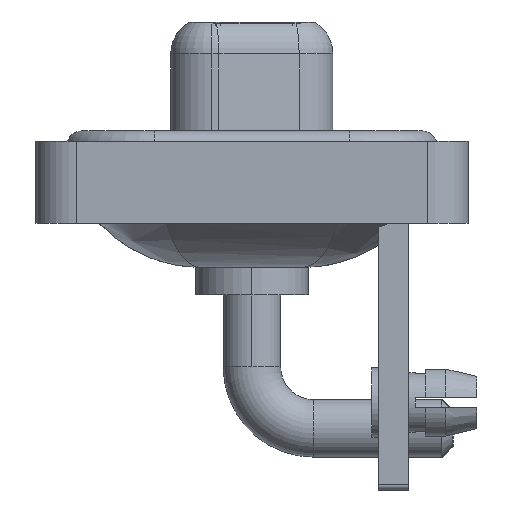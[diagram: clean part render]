
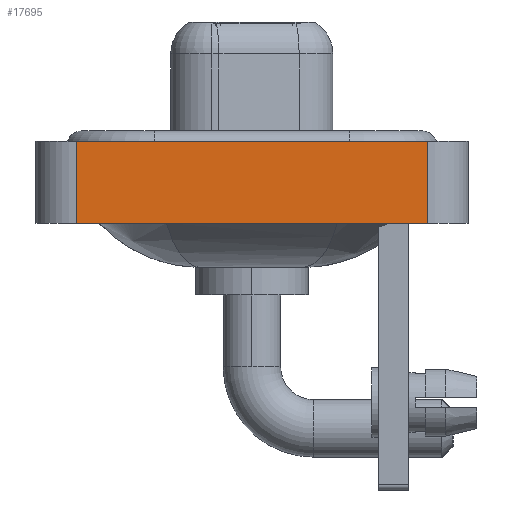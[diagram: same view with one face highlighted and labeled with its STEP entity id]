
A CAD part, left-side view. The second image highlights one B-rep face of the part: STEP entity #17695.
In plain terms, the highlighted planar face has unit normal (-1, 0, 0).
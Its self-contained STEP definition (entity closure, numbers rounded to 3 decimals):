
#284 = VERTEX_POINT ( 'NONE', #9182 ) ;
#681 = ORIENTED_EDGE ( 'NONE', *, *, #9010, .T. ) ;
#1089 = VERTEX_POINT ( 'NONE', #16234 ) ;
#1269 = VERTEX_POINT ( 'NONE', #14021 ) ;
#1744 = CARTESIAN_POINT ( 'NONE',  ( -7.3, 8.55, -3.6 ) ) ;
#1840 = ORIENTED_EDGE ( 'NONE', *, *, #10058, .F. ) ;
#1850 = EDGE_CURVE ( 'NONE', #13147, #1089, #11886, .T. ) ;
#1925 = LINE ( 'NONE', #2033, #12495 ) ;
#2018 = LINE ( 'NONE', #9761, #18036 ) ;
#2033 = CARTESIAN_POINT ( 'NONE',  ( -7.3, -8.55, -3.6 ) ) ;
#2707 = FACE_OUTER_BOUND ( 'NONE', #12504, .T. ) ;
#2946 = ORIENTED_EDGE ( 'NONE', *, *, #1850, .T. ) ;
#3979 = LINE ( 'NONE', #10131, #13502 ) ;
#5917 = EDGE_CURVE ( 'NONE', #13147, #284, #2018, .T. ) ;
#6331 = AXIS2_PLACEMENT_3D ( 'NONE', #9953, #8554, #14588 ) ;
#8554 = DIRECTION ( 'NONE',  ( -1., 0., 0. ) ) ;
#9010 = EDGE_CURVE ( 'NONE', #1089, #1269, #1925, .T. ) ;
#9182 = CARTESIAN_POINT ( 'NONE',  ( -7.3, 8.55, 0.4 ) ) ;
#9761 = CARTESIAN_POINT ( 'NONE',  ( -7.3, 8.55, -3.6 ) ) ;
#9953 = CARTESIAN_POINT ( 'NONE',  ( -7.3, -8.55, -3.6 ) ) ;
#9983 = CARTESIAN_POINT ( 'NONE',  ( -7.3, -8.55, -3.6 ) ) ;
#10058 = EDGE_CURVE ( 'NONE', #284, #1269, #3979, .T. ) ;
#10131 = CARTESIAN_POINT ( 'NONE',  ( -7.3, -8.55, 0.4 ) ) ;
#11886 = LINE ( 'NONE', #9983, #13329 ) ;
#12495 = VECTOR ( 'NONE', #16001, 1000. ) ;
#12504 = EDGE_LOOP ( 'NONE', ( #681, #1840, #15958, #2946 ) ) ;
#13147 = VERTEX_POINT ( 'NONE', #1744 ) ;
#13329 = VECTOR ( 'NONE', #18524, 1000. ) ;
#13355 = DIRECTION ( 'NONE',  ( 0., -1., 0. ) ) ;
#13502 = VECTOR ( 'NONE', #13355, 1000. ) ;
#14021 = CARTESIAN_POINT ( 'NONE',  ( -7.3, -8.55, 0.4 ) ) ;
#14588 = DIRECTION ( 'NONE',  ( 0., 0., 1. ) ) ;
#15958 = ORIENTED_EDGE ( 'NONE', *, *, #5917, .F. ) ;
#16001 = DIRECTION ( 'NONE',  ( 0., 0., 1. ) ) ;
#16234 = CARTESIAN_POINT ( 'NONE',  ( -7.3, -8.55, -3.6 ) ) ;
#17695 = ADVANCED_FACE ( 'NONE', ( #2707 ), #19410, .T. ) ;
#18036 = VECTOR ( 'NONE', #18812, 1000. ) ;
#18524 = DIRECTION ( 'NONE',  ( 0., -1., 0. ) ) ;
#18812 = DIRECTION ( 'NONE',  ( 0., 0., 1. ) ) ;
#19410 = PLANE ( 'NONE',  #6331 ) ;
